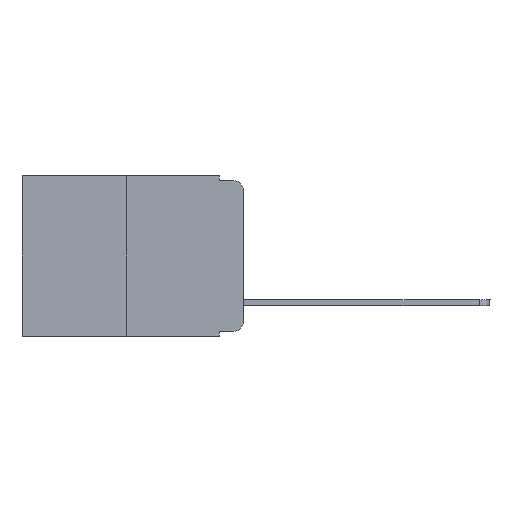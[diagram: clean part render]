
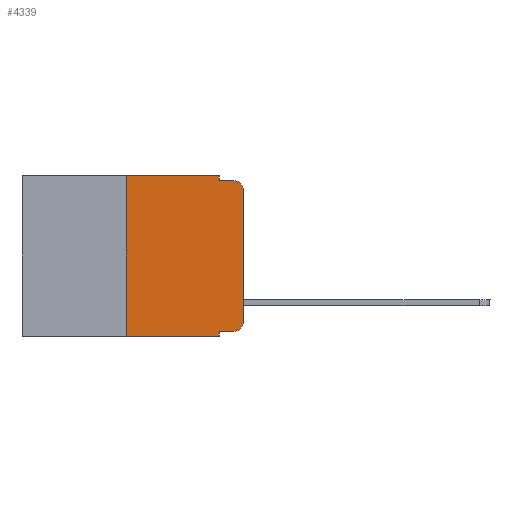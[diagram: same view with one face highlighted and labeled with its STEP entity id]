
A CAD part, left-side view. The second image highlights one B-rep face of the part: STEP entity #4339.
In plain terms, the highlighted planar face has unit normal (-1, 0, 0).
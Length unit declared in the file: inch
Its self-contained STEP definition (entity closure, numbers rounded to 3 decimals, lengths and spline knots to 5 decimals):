
#147 = CARTESIAN_POINT ( 'NONE',  ( 0., 0.051, -0.333 ) ) ;
#306 = ORIENTED_EDGE ( 'NONE', *, *, #7877, .T. ) ;
#371 = LINE ( 'NONE', #10532, #5621 ) ;
#516 = ORIENTED_EDGE ( 'NONE', *, *, #1230, .F. ) ;
#526 = CARTESIAN_POINT ( 'NONE',  ( 0., 0.25, 0. ) ) ;
#554 = AXIS2_PLACEMENT_3D ( 'NONE', #9341, #12377, #10441 ) ;
#851 = VERTEX_POINT ( 'NONE', #1434 ) ;
#856 = ORIENTED_EDGE ( 'NONE', *, *, #905, .T. ) ;
#905 = EDGE_CURVE ( 'NONE', #3796, #4994, #1775, .T. ) ;
#1163 = CARTESIAN_POINT ( 'NONE',  ( 0., 0.051, 0. ) ) ;
#1230 = EDGE_CURVE ( 'NONE', #851, #11447, #7373, .T. ) ;
#1359 = CARTESIAN_POINT ( 'NONE',  ( 0., 0.02, -0.313 ) ) ;
#1434 = CARTESIAN_POINT ( 'NONE',  ( 0., 0.051, -0.333 ) ) ;
#1677 = LINE ( 'NONE', #3514, #12593 ) ;
#1775 = LINE ( 'NONE', #3686, #9031 ) ;
#1889 = DIRECTION ( 'NONE',  ( 1., 0., 0. ) ) ;
#1977 = VERTEX_POINT ( 'NONE', #6615 ) ;
#3038 = VECTOR ( 'NONE', #7954, 39.37008 ) ;
#3242 = LINE ( 'NONE', #147, #10692 ) ;
#3514 = CARTESIAN_POINT ( 'NONE',  ( 0., 0.051, 0. ) ) ;
#3630 = CARTESIAN_POINT ( 'NONE',  ( 0., 0., -0.03 ) ) ;
#3686 = CARTESIAN_POINT ( 'NONE',  ( 0., 0., 0. ) ) ;
#3763 = CARTESIAN_POINT ( 'NONE',  ( 0., 0.051, -0.343 ) ) ;
#3772 = EDGE_CURVE ( 'NONE', #1977, #12919, #1677, .T. ) ;
#3796 = VERTEX_POINT ( 'NONE', #10112 ) ;
#3912 = VECTOR ( 'NONE', #5692, 39.37008 ) ;
#4056 = AXIS2_PLACEMENT_3D ( 'NONE', #1359, #4513, #10932 ) ;
#4079 = VERTEX_POINT ( 'NONE', #526 ) ;
#4296 = CIRCLE ( 'NONE', #4056, 0.02 ) ;
#4339 = ADVANCED_FACE ( 'NONE', ( #9400 ), #6803, .F. ) ;
#4364 = CARTESIAN_POINT ( 'NONE',  ( 0., 0.25, 0. ) ) ;
#4513 = DIRECTION ( 'NONE',  ( -1., 0., 0. ) ) ;
#4631 = LINE ( 'NONE', #7830, #11118 ) ;
#4773 = DIRECTION ( 'NONE',  ( 0., 0., 1. ) ) ;
#4813 = VERTEX_POINT ( 'NONE', #9785 ) ;
#4994 = VERTEX_POINT ( 'NONE', #3630 ) ;
#5547 = VECTOR ( 'NONE', #13287, 39.37008 ) ;
#5621 = VECTOR ( 'NONE', #11602, 39.37008 ) ;
#5692 = DIRECTION ( 'NONE',  ( 0., 0., 1. ) ) ;
#5745 = CARTESIAN_POINT ( 'NONE',  ( 0., 0.02, -0.333 ) ) ;
#5903 = ORIENTED_EDGE ( 'NONE', *, *, #3772, .F. ) ;
#6132 = EDGE_CURVE ( 'NONE', #851, #7617, #3242, .T. ) ;
#6388 = CARTESIAN_POINT ( 'NONE',  ( 0., 0.051, -0.01 ) ) ;
#6536 = ORIENTED_EDGE ( 'NONE', *, *, #6132, .T. ) ;
#6615 = CARTESIAN_POINT ( 'NONE',  ( 0., 0.051, 0. ) ) ;
#6803 = PLANE ( 'NONE',  #8262 ) ;
#7158 = VERTEX_POINT ( 'NONE', #11344 ) ;
#7373 = LINE ( 'NONE', #1163, #5547 ) ;
#7505 = DIRECTION ( 'NONE',  ( 0., -1., 0. ) ) ;
#7617 = VERTEX_POINT ( 'NONE', #5745 ) ;
#7830 = CARTESIAN_POINT ( 'NONE',  ( 0., 0.051, -0.01 ) ) ;
#7845 = CARTESIAN_POINT ( 'NONE',  ( 0., 0.473, -0.343 ) ) ;
#7877 = EDGE_CURVE ( 'NONE', #4994, #7158, #9952, .T. ) ;
#7954 = DIRECTION ( 'NONE',  ( 0., -1., 0. ) ) ;
#8262 = AXIS2_PLACEMENT_3D ( 'NONE', #13334, #1889, #12470 ) ;
#8461 = LINE ( 'NONE', #7845, #3038 ) ;
#8521 = ORIENTED_EDGE ( 'NONE', *, *, #12626, .T. ) ;
#8739 = EDGE_CURVE ( 'NONE', #7617, #3796, #4296, .T. ) ;
#8902 = DIRECTION ( 'NONE',  ( 0., 0., -1. ) ) ;
#9031 = VECTOR ( 'NONE', #4773, 39.37008 ) ;
#9341 = CARTESIAN_POINT ( 'NONE',  ( 0., 0.02, -0.03 ) ) ;
#9400 = FACE_OUTER_BOUND ( 'NONE', #13612, .T. ) ;
#9602 = ORIENTED_EDGE ( 'NONE', *, *, #9605, .F. ) ;
#9605 = EDGE_CURVE ( 'NONE', #4079, #1977, #371, .T. ) ;
#9785 = CARTESIAN_POINT ( 'NONE',  ( 0., 0.25, -0.343 ) ) ;
#9952 = CIRCLE ( 'NONE', #554, 0.02 ) ;
#10112 = CARTESIAN_POINT ( 'NONE',  ( 0., 0., -0.313 ) ) ;
#10441 = DIRECTION ( 'NONE',  ( 0., 0., -1. ) ) ;
#10532 = CARTESIAN_POINT ( 'NONE',  ( 0., 0.473, 0. ) ) ;
#10692 = VECTOR ( 'NONE', #7505, 39.37008 ) ;
#10932 = DIRECTION ( 'NONE',  ( 0., 0., -1. ) ) ;
#11118 = VECTOR ( 'NONE', #11995, 39.37008 ) ;
#11177 = EDGE_CURVE ( 'NONE', #4813, #4079, #12715, .T. ) ;
#11311 = ORIENTED_EDGE ( 'NONE', *, *, #13215, .F. ) ;
#11344 = CARTESIAN_POINT ( 'NONE',  ( 0., 0.02, -0.01 ) ) ;
#11447 = VERTEX_POINT ( 'NONE', #3763 ) ;
#11602 = DIRECTION ( 'NONE',  ( 0., -1., 0. ) ) ;
#11995 = DIRECTION ( 'NONE',  ( 0., -1., 0. ) ) ;
#12377 = DIRECTION ( 'NONE',  ( -1., 0., 0. ) ) ;
#12470 = DIRECTION ( 'NONE',  ( 0., 0., -1. ) ) ;
#12593 = VECTOR ( 'NONE', #8902, 39.37008 ) ;
#12626 = EDGE_CURVE ( 'NONE', #4813, #11447, #8461, .T. ) ;
#12715 = LINE ( 'NONE', #4364, #3912 ) ;
#12817 = ORIENTED_EDGE ( 'NONE', *, *, #11177, .F. ) ;
#12919 = VERTEX_POINT ( 'NONE', #6388 ) ;
#13215 = EDGE_CURVE ( 'NONE', #12919, #7158, #4631, .T. ) ;
#13287 = DIRECTION ( 'NONE',  ( 0., 0., -1. ) ) ;
#13334 = CARTESIAN_POINT ( 'NONE',  ( 0., 0.473, 0. ) ) ;
#13529 = ORIENTED_EDGE ( 'NONE', *, *, #8739, .T. ) ;
#13612 = EDGE_LOOP ( 'NONE', ( #856, #306, #11311, #5903, #9602, #12817, #8521, #516, #6536, #13529 ) ) ;
